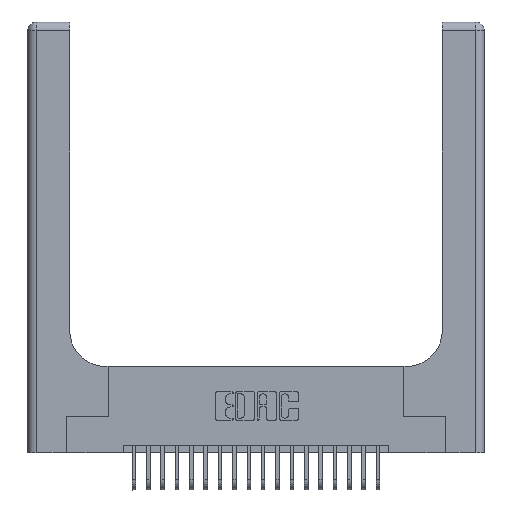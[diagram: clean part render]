
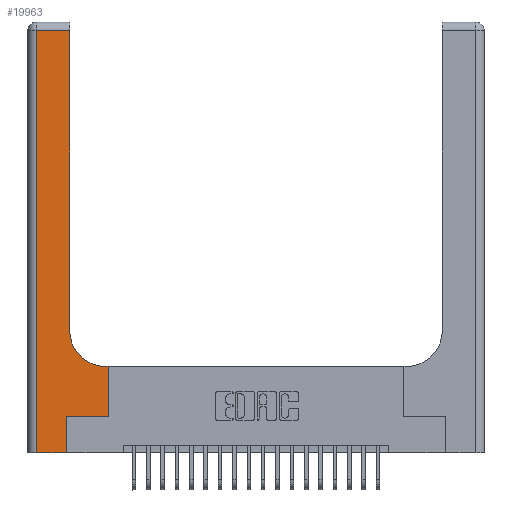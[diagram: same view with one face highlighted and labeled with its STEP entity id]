
A CAD part, top view. The second image highlights one B-rep face of the part: STEP entity #19963.
In plain terms, the highlighted planar face has unit normal (0, 0, 1).
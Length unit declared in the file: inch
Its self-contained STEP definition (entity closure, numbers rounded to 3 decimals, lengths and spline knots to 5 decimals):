
#23 = VECTOR ( 'NONE', #1256, 39.37008 ) ;
#452 = FACE_OUTER_BOUND ( 'NONE', #5074, .T. ) ;
#649 = EDGE_CURVE ( 'NONE', #2054, #20858, #18253, .T. ) ;
#722 = VERTEX_POINT ( 'NONE', #8794 ) ;
#1201 = DIRECTION ( 'NONE',  ( 1., 0., 0. ) ) ;
#1256 = DIRECTION ( 'NONE',  ( 0., -1., 0. ) ) ;
#1473 = VECTOR ( 'NONE', #16791, 39.37008 ) ;
#2054 = VERTEX_POINT ( 'NONE', #20870 ) ;
#2058 = CARTESIAN_POINT ( 'NONE',  ( 0., 3., 0.37 ) ) ;
#2552 = LINE ( 'NONE', #4905, #1473 ) ;
#2690 = EDGE_CURVE ( 'NONE', #8116, #21513, #9192, .T. ) ;
#2850 = CARTESIAN_POINT ( 'NONE',  ( 0.06, 3., 0.37 ) ) ;
#3482 = CARTESIAN_POINT ( 'NONE',  ( 0.269, 0., 0.37 ) ) ;
#3719 = DIRECTION ( 'NONE',  ( 1., 0., 0. ) ) ;
#4224 = CARTESIAN_POINT ( 'NONE',  ( 0.269, 0.25, 0.37 ) ) ;
#4273 = CARTESIAN_POINT ( 'NONE',  ( 0.2915, 2.94, 0.37 ) ) ;
#4301 = VERTEX_POINT ( 'NONE', #4224 ) ;
#4905 = CARTESIAN_POINT ( 'NONE',  ( 0., 2.94, 0.37 ) ) ;
#5001 = CARTESIAN_POINT ( 'NONE',  ( 0.06, 0., 0.37 ) ) ;
#5074 = EDGE_LOOP ( 'NONE', ( #18879, #6380, #12582, #8551, #18112, #20189, #20724, #8279, #11223 ) ) ;
#5206 = DIRECTION ( 'NONE',  ( 0., 1., 0. ) ) ;
#5432 = DIRECTION ( 'NONE',  ( -1., 0., 0. ) ) ;
#5562 = EDGE_CURVE ( 'NONE', #15346, #7410, #15942, .T. ) ;
#5772 = AXIS2_PLACEMENT_3D ( 'NONE', #21567, #11498, #1201 ) ;
#6324 = VECTOR ( 'NONE', #9647, 39.37008 ) ;
#6380 = ORIENTED_EDGE ( 'NONE', *, *, #11306, .T. ) ;
#6584 = CARTESIAN_POINT ( 'NONE',  ( 0.06, 2.94, 0.37 ) ) ;
#7111 = DIRECTION ( 'NONE',  ( 0., 1., 0. ) ) ;
#7217 = PLANE ( 'NONE',  #12997 ) ;
#7267 = VECTOR ( 'NONE', #18133, 39.37008 ) ;
#7410 = VERTEX_POINT ( 'NONE', #14822 ) ;
#7580 = EDGE_CURVE ( 'NONE', #722, #4301, #21854, .T. ) ;
#7685 = LINE ( 'NONE', #20687, #20665 ) ;
#8116 = VERTEX_POINT ( 'NONE', #6584 ) ;
#8279 = ORIENTED_EDGE ( 'NONE', *, *, #14808, .T. ) ;
#8551 = ORIENTED_EDGE ( 'NONE', *, *, #21649, .T. ) ;
#8794 = CARTESIAN_POINT ( 'NONE',  ( 0.269, 0., 0.37 ) ) ;
#8841 = CARTESIAN_POINT ( 'NONE',  ( 0.5415, 0.6, 0.37 ) ) ;
#8961 = DIRECTION ( 'NONE',  ( 0., 0., -1. ) ) ;
#9192 = LINE ( 'NONE', #2850, #23 ) ;
#9248 = LINE ( 'NONE', #15590, #17707 ) ;
#9261 = VECTOR ( 'NONE', #5206, 39.37008 ) ;
#9647 = DIRECTION ( 'NONE',  ( 1., 0., 0. ) ) ;
#11223 = ORIENTED_EDGE ( 'NONE', *, *, #5562, .T. ) ;
#11306 = EDGE_CURVE ( 'NONE', #13925, #8116, #2552, .T. ) ;
#11498 = DIRECTION ( 'NONE',  ( 0., 0., -1. ) ) ;
#12066 = EDGE_CURVE ( 'NONE', #7410, #13925, #9248, .T. ) ;
#12508 = LINE ( 'NONE', #13967, #21427 ) ;
#12582 = ORIENTED_EDGE ( 'NONE', *, *, #2690, .T. ) ;
#12997 = AXIS2_PLACEMENT_3D ( 'NONE', #2058, #8961, #20768 ) ;
#13925 = VERTEX_POINT ( 'NONE', #4273 ) ;
#13967 = CARTESIAN_POINT ( 'NONE',  ( 0., 0., 0.37 ) ) ;
#14808 = EDGE_CURVE ( 'NONE', #20858, #15346, #7685, .T. ) ;
#14822 = CARTESIAN_POINT ( 'NONE',  ( 0.2915, 0.85, 0.37 ) ) ;
#15346 = VERTEX_POINT ( 'NONE', #8841 ) ;
#15392 = LINE ( 'NONE', #19750, #6324 ) ;
#15590 = CARTESIAN_POINT ( 'NONE',  ( 0.2915, 3., 0.37 ) ) ;
#15942 = CIRCLE ( 'NONE', #5772, 0.25 ) ;
#16761 = CARTESIAN_POINT ( 'NONE',  ( 0.5585, 0.6, 0.37 ) ) ;
#16791 = DIRECTION ( 'NONE',  ( -1., 0., 0. ) ) ;
#17707 = VECTOR ( 'NONE', #7111, 39.37008 ) ;
#18112 = ORIENTED_EDGE ( 'NONE', *, *, #7580, .T. ) ;
#18133 = DIRECTION ( 'NONE',  ( 0., 1., 0. ) ) ;
#18253 = LINE ( 'NONE', #20395, #9261 ) ;
#18879 = ORIENTED_EDGE ( 'NONE', *, *, #12066, .T. ) ;
#19750 = CARTESIAN_POINT ( 'NONE',  ( 0.269, 0.25, 0.37 ) ) ;
#19963 = ADVANCED_FACE ( 'NONE', ( #452 ), #7217, .F. ) ;
#20189 = ORIENTED_EDGE ( 'NONE', *, *, #21302, .T. ) ;
#20395 = CARTESIAN_POINT ( 'NONE',  ( 0.5585, 0.25, 0.37 ) ) ;
#20665 = VECTOR ( 'NONE', #5432, 39.37008 ) ;
#20687 = CARTESIAN_POINT ( 'NONE',  ( 0.2915, 0.6, 0.37 ) ) ;
#20724 = ORIENTED_EDGE ( 'NONE', *, *, #649, .T. ) ;
#20768 = DIRECTION ( 'NONE',  ( -1., 0., 0. ) ) ;
#20858 = VERTEX_POINT ( 'NONE', #16761 ) ;
#20870 = CARTESIAN_POINT ( 'NONE',  ( 0.5585, 0.25, 0.37 ) ) ;
#21302 = EDGE_CURVE ( 'NONE', #4301, #2054, #15392, .T. ) ;
#21427 = VECTOR ( 'NONE', #3719, 39.37008 ) ;
#21513 = VERTEX_POINT ( 'NONE', #5001 ) ;
#21567 = CARTESIAN_POINT ( 'NONE',  ( 0.5415, 0.85, 0.37 ) ) ;
#21649 = EDGE_CURVE ( 'NONE', #21513, #722, #12508, .T. ) ;
#21854 = LINE ( 'NONE', #3482, #7267 ) ;
